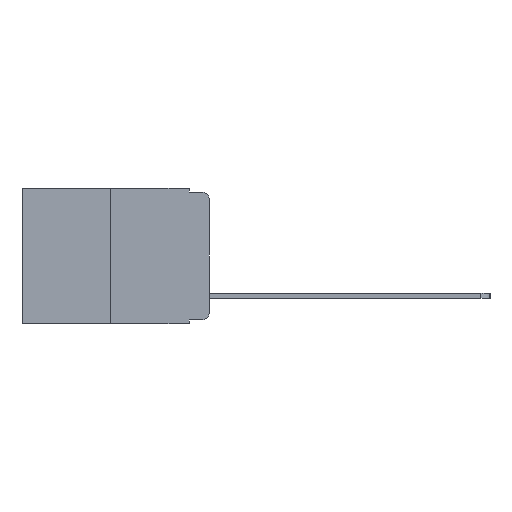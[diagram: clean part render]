
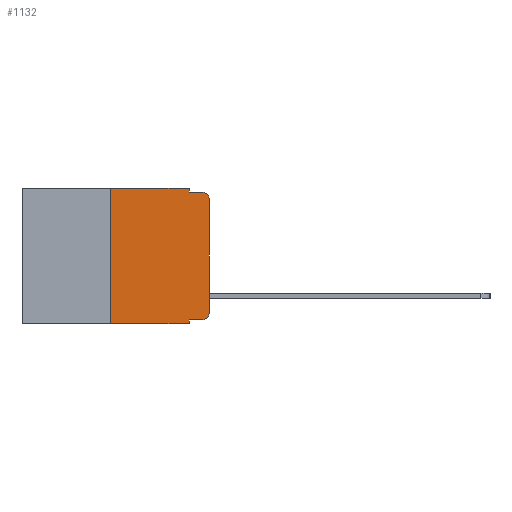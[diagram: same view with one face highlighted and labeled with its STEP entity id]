
A CAD part, left-side view. The second image highlights one B-rep face of the part: STEP entity #1132.
In plain terms, the highlighted planar face has unit normal (-1, 0, 0).
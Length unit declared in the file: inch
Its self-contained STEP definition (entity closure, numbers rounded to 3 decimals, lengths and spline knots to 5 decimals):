
#125 = DIRECTION ( 'NONE',  ( 0., 0., -1. ) ) ;
#191 = DIRECTION ( 'NONE',  ( 0., 0., 1. ) ) ;
#226 = CARTESIAN_POINT ( 'NONE',  ( 0., 0.051, 0. ) ) ;
#250 = DIRECTION ( 'NONE',  ( -1., 0., 0. ) ) ;
#591 = CARTESIAN_POINT ( 'NONE',  ( 0., 0.051, -0.343 ) ) ;
#672 = CARTESIAN_POINT ( 'NONE',  ( 0., 0.25, -0.343 ) ) ;
#850 = PLANE ( 'NONE',  #7612 ) ;
#851 = DIRECTION ( 'NONE',  ( 0., 0., -1. ) ) ;
#889 = CARTESIAN_POINT ( 'NONE',  ( 0., 0.051, 0. ) ) ;
#1025 = LINE ( 'NONE', #4309, #8082 ) ;
#1088 = VERTEX_POINT ( 'NONE', #6305 ) ;
#1111 = AXIS2_PLACEMENT_3D ( 'NONE', #7351, #250, #1708 ) ;
#1132 = ADVANCED_FACE ( 'NONE', ( #8230 ), #850, .F. ) ;
#1435 = CARTESIAN_POINT ( 'NONE',  ( 0., 0.473, 0. ) ) ;
#1708 = DIRECTION ( 'NONE',  ( 0., 0., -1. ) ) ;
#1811 = DIRECTION ( 'NONE',  ( 1., 0., 0. ) ) ;
#1829 = CARTESIAN_POINT ( 'NONE',  ( 0., 0., -0.313 ) ) ;
#1931 = VERTEX_POINT ( 'NONE', #1829 ) ;
#1968 = VECTOR ( 'NONE', #851, 39.37008 ) ;
#2648 = EDGE_CURVE ( 'NONE', #7694, #5116, #6725, .T. ) ;
#2827 = LINE ( 'NONE', #5831, #9413 ) ;
#2840 = CARTESIAN_POINT ( 'NONE',  ( 0., 0.25, 0. ) ) ;
#3536 = ORIENTED_EDGE ( 'NONE', *, *, #4694, .T. ) ;
#3717 = EDGE_CURVE ( 'NONE', #10216, #9695, #7722, .T. ) ;
#3720 = VECTOR ( 'NONE', #125, 39.37008 ) ;
#4297 = EDGE_CURVE ( 'NONE', #8745, #10016, #2827, .T. ) ;
#4309 = CARTESIAN_POINT ( 'NONE',  ( 0., 0.051, -0.333 ) ) ;
#4349 = DIRECTION ( 'NONE',  ( 0., 0., -1. ) ) ;
#4434 = VECTOR ( 'NONE', #6671, 39.37008 ) ;
#4465 = ORIENTED_EDGE ( 'NONE', *, *, #2648, .F. ) ;
#4694 = EDGE_CURVE ( 'NONE', #10647, #1088, #1025, .T. ) ;
#5051 = ORIENTED_EDGE ( 'NONE', *, *, #9037, .F. ) ;
#5067 = DIRECTION ( 'NONE',  ( -1., 0., 0. ) ) ;
#5104 = AXIS2_PLACEMENT_3D ( 'NONE', #9851, #5067, #10620 ) ;
#5116 = VERTEX_POINT ( 'NONE', #6356 ) ;
#5487 = CARTESIAN_POINT ( 'NONE',  ( 0., 0., -0.03 ) ) ;
#5624 = DIRECTION ( 'NONE',  ( 0., -1., 0. ) ) ;
#5777 = ORIENTED_EDGE ( 'NONE', *, *, #6920, .F. ) ;
#5831 = CARTESIAN_POINT ( 'NONE',  ( 0., 0.473, -0.343 ) ) ;
#6092 = ORIENTED_EDGE ( 'NONE', *, *, #10041, .F. ) ;
#6166 = LINE ( 'NONE', #226, #3720 ) ;
#6167 = DIRECTION ( 'NONE',  ( 0., 0., 1. ) ) ;
#6180 = EDGE_CURVE ( 'NONE', #1931, #10216, #6298, .T. ) ;
#6298 = LINE ( 'NONE', #6938, #8184 ) ;
#6305 = CARTESIAN_POINT ( 'NONE',  ( 0., 0.02, -0.333 ) ) ;
#6356 = CARTESIAN_POINT ( 'NONE',  ( 0., 0.051, 0. ) ) ;
#6636 = ORIENTED_EDGE ( 'NONE', *, *, #6988, .F. ) ;
#6671 = DIRECTION ( 'NONE',  ( 0., -1., 0. ) ) ;
#6693 = VECTOR ( 'NONE', #191, 39.37008 ) ;
#6725 = LINE ( 'NONE', #10208, #4434 ) ;
#6920 = EDGE_CURVE ( 'NONE', #5116, #8916, #8778, .T. ) ;
#6938 = CARTESIAN_POINT ( 'NONE',  ( 0., 0., 0. ) ) ;
#6988 = EDGE_CURVE ( 'NONE', #10647, #10016, #6166, .T. ) ;
#7351 = CARTESIAN_POINT ( 'NONE',  ( 0., 0.02, -0.03 ) ) ;
#7409 = DIRECTION ( 'NONE',  ( 0., -1., 0. ) ) ;
#7612 = AXIS2_PLACEMENT_3D ( 'NONE', #1435, #1811, #4349 ) ;
#7694 = VERTEX_POINT ( 'NONE', #2840 ) ;
#7722 = CIRCLE ( 'NONE', #1111, 0.02 ) ;
#7942 = VECTOR ( 'NONE', #8056, 39.37008 ) ;
#8056 = DIRECTION ( 'NONE',  ( 0., -1., 0. ) ) ;
#8082 = VECTOR ( 'NONE', #7409, 39.37008 ) ;
#8184 = VECTOR ( 'NONE', #6167, 39.37008 ) ;
#8230 = FACE_OUTER_BOUND ( 'NONE', #9684, .T. ) ;
#8745 = VERTEX_POINT ( 'NONE', #672 ) ;
#8778 = LINE ( 'NONE', #889, #1968 ) ;
#8817 = LINE ( 'NONE', #10722, #6693 ) ;
#8876 = ORIENTED_EDGE ( 'NONE', *, *, #4297, .T. ) ;
#8916 = VERTEX_POINT ( 'NONE', #9124 ) ;
#8942 = ORIENTED_EDGE ( 'NONE', *, *, #6180, .T. ) ;
#9037 = EDGE_CURVE ( 'NONE', #8745, #7694, #8817, .T. ) ;
#9124 = CARTESIAN_POINT ( 'NONE',  ( 0., 0.051, -0.01 ) ) ;
#9216 = CARTESIAN_POINT ( 'NONE',  ( 0., 0.051, -0.333 ) ) ;
#9350 = ORIENTED_EDGE ( 'NONE', *, *, #3717, .T. ) ;
#9401 = CIRCLE ( 'NONE', #5104, 0.02 ) ;
#9413 = VECTOR ( 'NONE', #5624, 39.37008 ) ;
#9616 = EDGE_CURVE ( 'NONE', #1088, #1931, #9401, .T. ) ;
#9684 = EDGE_LOOP ( 'NONE', ( #8942, #9350, #6092, #5777, #4465, #5051, #8876, #6636, #3536, #9740 ) ) ;
#9695 = VERTEX_POINT ( 'NONE', #9922 ) ;
#9740 = ORIENTED_EDGE ( 'NONE', *, *, #9616, .T. ) ;
#9851 = CARTESIAN_POINT ( 'NONE',  ( 0., 0.02, -0.313 ) ) ;
#9922 = CARTESIAN_POINT ( 'NONE',  ( 0., 0.02, -0.01 ) ) ;
#10016 = VERTEX_POINT ( 'NONE', #591 ) ;
#10041 = EDGE_CURVE ( 'NONE', #8916, #9695, #10443, .T. ) ;
#10208 = CARTESIAN_POINT ( 'NONE',  ( 0., 0.473, 0. ) ) ;
#10216 = VERTEX_POINT ( 'NONE', #5487 ) ;
#10443 = LINE ( 'NONE', #11054, #7942 ) ;
#10620 = DIRECTION ( 'NONE',  ( 0., 0., -1. ) ) ;
#10647 = VERTEX_POINT ( 'NONE', #9216 ) ;
#10722 = CARTESIAN_POINT ( 'NONE',  ( 0., 0.25, 0. ) ) ;
#11054 = CARTESIAN_POINT ( 'NONE',  ( 0., 0.051, -0.01 ) ) ;
